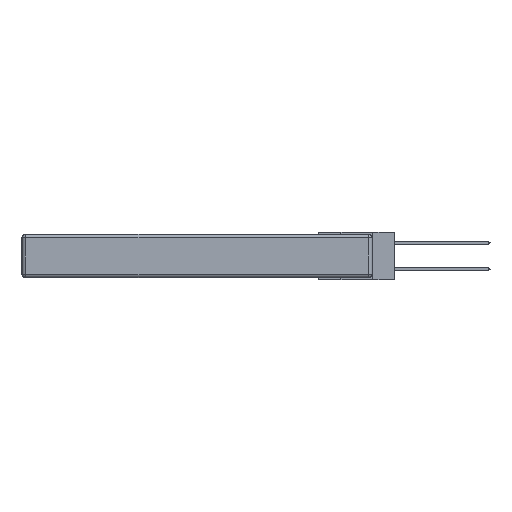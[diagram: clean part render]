
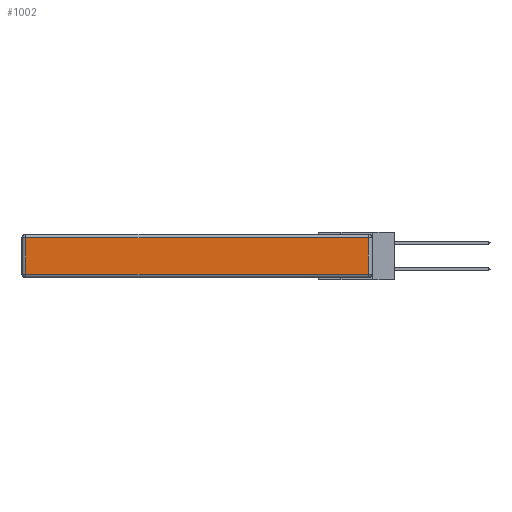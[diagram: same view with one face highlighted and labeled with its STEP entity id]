
A CAD part, left-side view. The second image highlights one B-rep face of the part: STEP entity #1002.
In plain terms, the highlighted planar face has unit normal (-1, 0, 0).
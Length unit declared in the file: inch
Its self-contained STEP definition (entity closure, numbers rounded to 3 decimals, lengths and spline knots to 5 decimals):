
#817 = EDGE_CURVE ( 'NONE', #22979, #7373, #14772, .T. ) ;
#1002 = ADVANCED_FACE ( 'NONE', ( #24361 ), #16552, .T. ) ;
#1173 = DIRECTION ( 'NONE',  ( -1., 0., 0. ) ) ;
#1267 = EDGE_CURVE ( 'NONE', #17814, #22979, #15029, .T. ) ;
#2115 = EDGE_LOOP ( 'NONE', ( #20725, #19121, #4196, #22516 ) ) ;
#3686 = CARTESIAN_POINT ( 'NONE',  ( 0., 0.03, -0.343 ) ) ;
#3713 = DIRECTION ( 'NONE',  ( 0., -1., 0. ) ) ;
#4196 = ORIENTED_EDGE ( 'NONE', *, *, #8077, .T. ) ;
#6869 = CARTESIAN_POINT ( 'NONE',  ( 0., 0., -0.343 ) ) ;
#7019 = DIRECTION ( 'NONE',  ( 0., 0., 1. ) ) ;
#7373 = VERTEX_POINT ( 'NONE', #23515 ) ;
#7560 = CARTESIAN_POINT ( 'NONE',  ( 0., 2.72, -0.343 ) ) ;
#8077 = EDGE_CURVE ( 'NONE', #7373, #20642, #21099, .T. ) ;
#8145 = DIRECTION ( 'NONE',  ( 0., 1., 0. ) ) ;
#9484 = DIRECTION ( 'NONE',  ( 0., 0., -1. ) ) ;
#11402 = CARTESIAN_POINT ( 'NONE',  ( 0., 2.72, -0.313 ) ) ;
#12639 = VECTOR ( 'NONE', #3713, 39.37008 ) ;
#12745 = CARTESIAN_POINT ( 'NONE',  ( 0., 0.03, -0.313 ) ) ;
#14772 = LINE ( 'NONE', #3686, #15357 ) ;
#14800 = AXIS2_PLACEMENT_3D ( 'NONE', #6869, #1173, #7019 ) ;
#15029 = LINE ( 'NONE', #15274, #12639 ) ;
#15274 = CARTESIAN_POINT ( 'NONE',  ( 0., 0., -0.313 ) ) ;
#15334 = DIRECTION ( 'NONE',  ( 0., 0., 1. ) ) ;
#15357 = VECTOR ( 'NONE', #15334, 39.37008 ) ;
#16552 = PLANE ( 'NONE',  #14800 ) ;
#17563 = VECTOR ( 'NONE', #9484, 39.37008 ) ;
#17678 = CARTESIAN_POINT ( 'NONE',  ( 0., 2.75, -0.03 ) ) ;
#17814 = VERTEX_POINT ( 'NONE', #11402 ) ;
#18794 = CARTESIAN_POINT ( 'NONE',  ( 0., 2.72, -0.03 ) ) ;
#19121 = ORIENTED_EDGE ( 'NONE', *, *, #817, .T. ) ;
#19659 = LINE ( 'NONE', #7560, #17563 ) ;
#20642 = VERTEX_POINT ( 'NONE', #18794 ) ;
#20725 = ORIENTED_EDGE ( 'NONE', *, *, #1267, .T. ) ;
#21099 = LINE ( 'NONE', #17678, #22583 ) ;
#22516 = ORIENTED_EDGE ( 'NONE', *, *, #24174, .T. ) ;
#22583 = VECTOR ( 'NONE', #8145, 39.37008 ) ;
#22979 = VERTEX_POINT ( 'NONE', #12745 ) ;
#23515 = CARTESIAN_POINT ( 'NONE',  ( 0., 0.03, -0.03 ) ) ;
#24174 = EDGE_CURVE ( 'NONE', #20642, #17814, #19659, .T. ) ;
#24361 = FACE_OUTER_BOUND ( 'NONE', #2115, .T. ) ;
